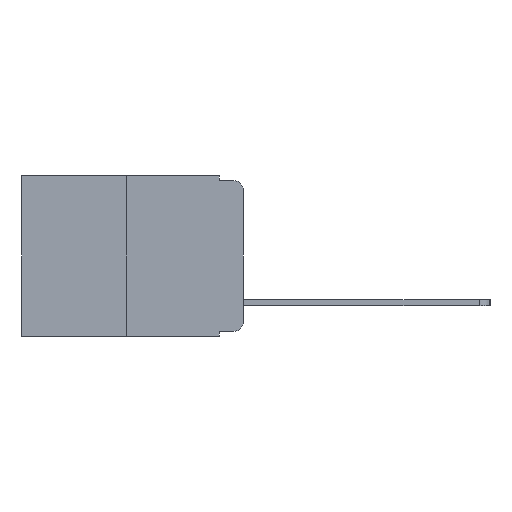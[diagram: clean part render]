
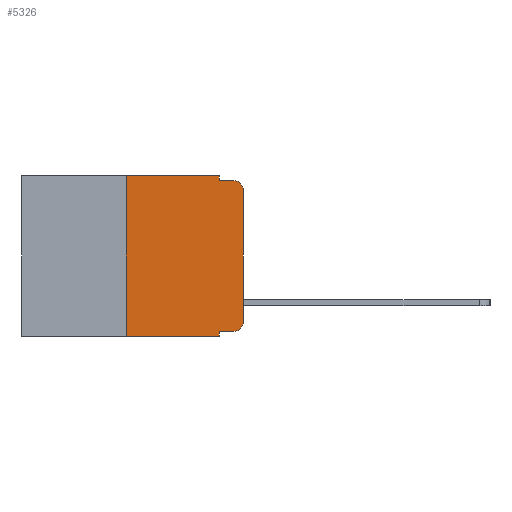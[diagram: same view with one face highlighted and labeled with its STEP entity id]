
A CAD part, left-side view. The second image highlights one B-rep face of the part: STEP entity #5326.
In plain terms, the highlighted planar face has unit normal (-1, 0, 0).
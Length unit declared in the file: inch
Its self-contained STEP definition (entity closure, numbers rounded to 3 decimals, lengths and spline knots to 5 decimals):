
#50 = EDGE_CURVE ( 'NONE', #573, #4084, #466, .T. ) ;
#453 = VECTOR ( 'NONE', #11834, 39.37008 ) ;
#466 = LINE ( 'NONE', #14827, #14789 ) ;
#573 = VERTEX_POINT ( 'NONE', #3693 ) ;
#818 = ORIENTED_EDGE ( 'NONE', *, *, #13433, .F. ) ;
#1347 = LINE ( 'NONE', #5180, #453 ) ;
#1505 = VERTEX_POINT ( 'NONE', #7883 ) ;
#1680 = DIRECTION ( 'NONE',  ( 0., 0., -1. ) ) ;
#1958 = VECTOR ( 'NONE', #8691, 39.37008 ) ;
#2001 = VERTEX_POINT ( 'NONE', #14768 ) ;
#2851 = CARTESIAN_POINT ( 'NONE',  ( 0., 0.473, -0.343 ) ) ;
#3116 = DIRECTION ( 'NONE',  ( 0., -1., 0. ) ) ;
#3259 = ORIENTED_EDGE ( 'NONE', *, *, #8954, .T. ) ;
#3534 = DIRECTION ( 'NONE',  ( -1., 0., 0. ) ) ;
#3693 = CARTESIAN_POINT ( 'NONE',  ( 0., 0.051, 0. ) ) ;
#4084 = VERTEX_POINT ( 'NONE', #14392 ) ;
#4346 = VECTOR ( 'NONE', #3116, 39.37008 ) ;
#4452 = LINE ( 'NONE', #2851, #7241 ) ;
#4525 = CARTESIAN_POINT ( 'NONE',  ( 0., 0.051, -0.333 ) ) ;
#4875 = DIRECTION ( 'NONE',  ( 1., 0., 0. ) ) ;
#5157 = CARTESIAN_POINT ( 'NONE',  ( 0., 0.25, 0. ) ) ;
#5180 = CARTESIAN_POINT ( 'NONE',  ( 0., 0.25, 0. ) ) ;
#5195 = CARTESIAN_POINT ( 'NONE',  ( 0., 0.02, -0.333 ) ) ;
#5292 = VECTOR ( 'NONE', #1680, 39.37008 ) ;
#5295 = CARTESIAN_POINT ( 'NONE',  ( 0., 0.473, 0. ) ) ;
#5326 = ADVANCED_FACE ( 'NONE', ( #15021 ), #10201, .F. ) ;
#5654 = LINE ( 'NONE', #7375, #1958 ) ;
#5756 = EDGE_CURVE ( 'NONE', #15616, #15669, #12788, .T. ) ;
#5902 = DIRECTION ( 'NONE',  ( -1., 0., 0. ) ) ;
#6100 = EDGE_CURVE ( 'NONE', #15616, #6423, #7959, .T. ) ;
#6278 = CIRCLE ( 'NONE', #12262, 0.02 ) ;
#6423 = VERTEX_POINT ( 'NONE', #5195 ) ;
#6551 = VECTOR ( 'NONE', #9280, 39.37008 ) ;
#6851 = ORIENTED_EDGE ( 'NONE', *, *, #14431, .T. ) ;
#6884 = CARTESIAN_POINT ( 'NONE',  ( 0., 0.051, -0.01 ) ) ;
#7241 = VECTOR ( 'NONE', #8313, 39.37008 ) ;
#7269 = ORIENTED_EDGE ( 'NONE', *, *, #8905, .F. ) ;
#7375 = CARTESIAN_POINT ( 'NONE',  ( 0., 0., 0. ) ) ;
#7505 = ORIENTED_EDGE ( 'NONE', *, *, #6100, .T. ) ;
#7883 = CARTESIAN_POINT ( 'NONE',  ( 0., 0.02, -0.01 ) ) ;
#7959 = LINE ( 'NONE', #11144, #4346 ) ;
#8055 = VECTOR ( 'NONE', #17375, 39.37008 ) ;
#8313 = DIRECTION ( 'NONE',  ( 0., -1., 0. ) ) ;
#8691 = DIRECTION ( 'NONE',  ( 0., 0., 1. ) ) ;
#8905 = EDGE_CURVE ( 'NONE', #4084, #1505, #11566, .T. ) ;
#8954 = EDGE_CURVE ( 'NONE', #2001, #15669, #4452, .T. ) ;
#9280 = DIRECTION ( 'NONE',  ( 0., -1., 0. ) ) ;
#9360 = EDGE_LOOP ( 'NONE', ( #6851, #13448, #7269, #11396, #11229, #818, #3259, #15295, #7505, #14893 ) ) ;
#9849 = CARTESIAN_POINT ( 'NONE',  ( 0., 0.051, 0. ) ) ;
#9982 = VERTEX_POINT ( 'NONE', #16924 ) ;
#10201 = PLANE ( 'NONE',  #12428 ) ;
#10483 = LINE ( 'NONE', #5295, #6551 ) ;
#11144 = CARTESIAN_POINT ( 'NONE',  ( 0., 0.051, -0.333 ) ) ;
#11229 = ORIENTED_EDGE ( 'NONE', *, *, #13480, .F. ) ;
#11396 = ORIENTED_EDGE ( 'NONE', *, *, #50, .F. ) ;
#11557 = CARTESIAN_POINT ( 'NONE',  ( 0., 0.02, -0.313 ) ) ;
#11566 = LINE ( 'NONE', #6884, #8055 ) ;
#11709 = AXIS2_PLACEMENT_3D ( 'NONE', #11557, #3534, #12882 ) ;
#11834 = DIRECTION ( 'NONE',  ( 0., 0., 1. ) ) ;
#11913 = CIRCLE ( 'NONE', #11709, 0.02 ) ;
#12262 = AXIS2_PLACEMENT_3D ( 'NONE', #13844, #5902, #15115 ) ;
#12428 = AXIS2_PLACEMENT_3D ( 'NONE', #12856, #4875, #14172 ) ;
#12615 = CARTESIAN_POINT ( 'NONE',  ( 0., 0., -0.313 ) ) ;
#12788 = LINE ( 'NONE', #9849, #5292 ) ;
#12856 = CARTESIAN_POINT ( 'NONE',  ( 0., 0.473, 0. ) ) ;
#12882 = DIRECTION ( 'NONE',  ( 0., 0., -1. ) ) ;
#13433 = EDGE_CURVE ( 'NONE', #2001, #14075, #1347, .T. ) ;
#13448 = ORIENTED_EDGE ( 'NONE', *, *, #15597, .T. ) ;
#13480 = EDGE_CURVE ( 'NONE', #14075, #573, #10483, .T. ) ;
#13844 = CARTESIAN_POINT ( 'NONE',  ( 0., 0.02, -0.03 ) ) ;
#14012 = CARTESIAN_POINT ( 'NONE',  ( 0., 0.051, -0.343 ) ) ;
#14075 = VERTEX_POINT ( 'NONE', #5157 ) ;
#14172 = DIRECTION ( 'NONE',  ( 0., 0., -1. ) ) ;
#14392 = CARTESIAN_POINT ( 'NONE',  ( 0., 0.051, -0.01 ) ) ;
#14431 = EDGE_CURVE ( 'NONE', #16748, #9982, #5654, .T. ) ;
#14472 = DIRECTION ( 'NONE',  ( 0., 0., -1. ) ) ;
#14768 = CARTESIAN_POINT ( 'NONE',  ( 0., 0.25, -0.343 ) ) ;
#14789 = VECTOR ( 'NONE', #14472, 39.37008 ) ;
#14827 = CARTESIAN_POINT ( 'NONE',  ( 0., 0.051, 0. ) ) ;
#14893 = ORIENTED_EDGE ( 'NONE', *, *, #15126, .T. ) ;
#15021 = FACE_OUTER_BOUND ( 'NONE', #9360, .T. ) ;
#15115 = DIRECTION ( 'NONE',  ( 0., 0., -1. ) ) ;
#15126 = EDGE_CURVE ( 'NONE', #6423, #16748, #11913, .T. ) ;
#15295 = ORIENTED_EDGE ( 'NONE', *, *, #5756, .F. ) ;
#15597 = EDGE_CURVE ( 'NONE', #9982, #1505, #6278, .T. ) ;
#15616 = VERTEX_POINT ( 'NONE', #4525 ) ;
#15669 = VERTEX_POINT ( 'NONE', #14012 ) ;
#16748 = VERTEX_POINT ( 'NONE', #12615 ) ;
#16924 = CARTESIAN_POINT ( 'NONE',  ( 0., 0., -0.03 ) ) ;
#17375 = DIRECTION ( 'NONE',  ( 0., -1., 0. ) ) ;
